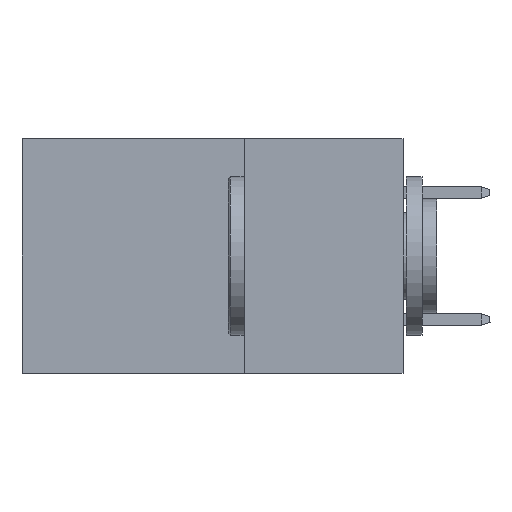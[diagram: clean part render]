
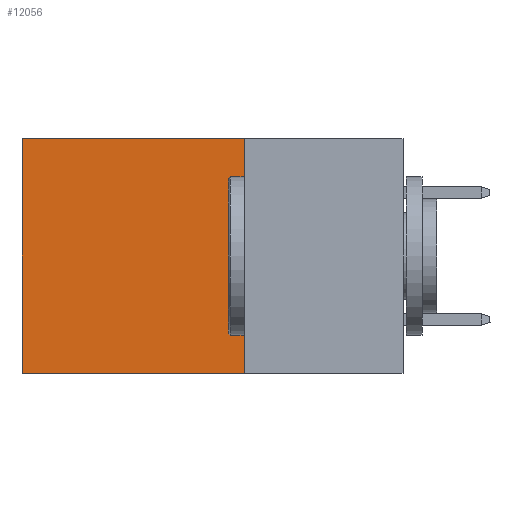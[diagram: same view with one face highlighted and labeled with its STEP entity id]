
A CAD part, left-side view. The second image highlights one B-rep face of the part: STEP entity #12056.
In plain terms, the highlighted planar face has unit normal (-1, 0, 0).
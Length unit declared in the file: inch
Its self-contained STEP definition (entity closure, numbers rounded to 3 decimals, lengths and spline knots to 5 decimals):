
#645 = EDGE_CURVE ( 'NONE', #6180, #5257, #1024, .T. ) ;
#846 = CARTESIAN_POINT ( 'NONE',  ( 0.2875, 0.25, -0.37 ) ) ;
#953 = DIRECTION ( 'NONE',  ( 0., 0., -1. ) ) ;
#1024 = LINE ( 'NONE', #5078, #14606 ) ;
#1177 = LINE ( 'NONE', #17320, #9460 ) ;
#1317 = CARTESIAN_POINT ( 'NONE',  ( 0.2875, 0.6, -0.37 ) ) ;
#2283 = PLANE ( 'NONE',  #11663 ) ;
#3490 = DIRECTION ( 'NONE',  ( 0., 1., 0. ) ) ;
#5020 = ORIENTED_EDGE ( 'NONE', *, *, #15284, .T. ) ;
#5078 = CARTESIAN_POINT ( 'NONE',  ( 0.2875, 0.25, 0. ) ) ;
#5257 = VERTEX_POINT ( 'NONE', #6726 ) ;
#6180 = VERTEX_POINT ( 'NONE', #15392 ) ;
#6422 = CARTESIAN_POINT ( 'NONE',  ( 0.2875, 0.6, 0. ) ) ;
#6726 = CARTESIAN_POINT ( 'NONE',  ( 0.2875, 0.6, 0. ) ) ;
#7376 = VECTOR ( 'NONE', #15852, 39.37008 ) ;
#7406 = FACE_OUTER_BOUND ( 'NONE', #9423, .T. ) ;
#7530 = ORIENTED_EDGE ( 'NONE', *, *, #645, .T. ) ;
#7664 = DIRECTION ( 'NONE',  ( 1., 0., 0. ) ) ;
#8796 = VERTEX_POINT ( 'NONE', #14753 ) ;
#9080 = CARTESIAN_POINT ( 'NONE',  ( 0.2875, 0.25, 0. ) ) ;
#9423 = EDGE_LOOP ( 'NONE', ( #5020, #16260, #13736, #7530 ) ) ;
#9460 = VECTOR ( 'NONE', #9716, 39.37008 ) ;
#9601 = EDGE_CURVE ( 'NONE', #8796, #13080, #17338, .T. ) ;
#9716 = DIRECTION ( 'NONE',  ( 0., 0., -1. ) ) ;
#10321 = VECTOR ( 'NONE', #17017, 39.37008 ) ;
#11663 = AXIS2_PLACEMENT_3D ( 'NONE', #9080, #7664, #953 ) ;
#12056 = ADVANCED_FACE ( 'NONE', ( #7406 ), #2283, .F. ) ;
#13080 = VERTEX_POINT ( 'NONE', #1317 ) ;
#13136 = LINE ( 'NONE', #6422, #10321 ) ;
#13736 = ORIENTED_EDGE ( 'NONE', *, *, #14449, .F. ) ;
#14449 = EDGE_CURVE ( 'NONE', #6180, #8796, #1177, .T. ) ;
#14606 = VECTOR ( 'NONE', #3490, 39.37008 ) ;
#14753 = CARTESIAN_POINT ( 'NONE',  ( 0.2875, 0.25, -0.37 ) ) ;
#15284 = EDGE_CURVE ( 'NONE', #5257, #13080, #13136, .T. ) ;
#15392 = CARTESIAN_POINT ( 'NONE',  ( 0.2875, 0.25, 0. ) ) ;
#15852 = DIRECTION ( 'NONE',  ( 0., 1., 0. ) ) ;
#16260 = ORIENTED_EDGE ( 'NONE', *, *, #9601, .F. ) ;
#17017 = DIRECTION ( 'NONE',  ( 0., 0., -1. ) ) ;
#17320 = CARTESIAN_POINT ( 'NONE',  ( 0.2875, 0.25, 0. ) ) ;
#17338 = LINE ( 'NONE', #846, #7376 ) ;
